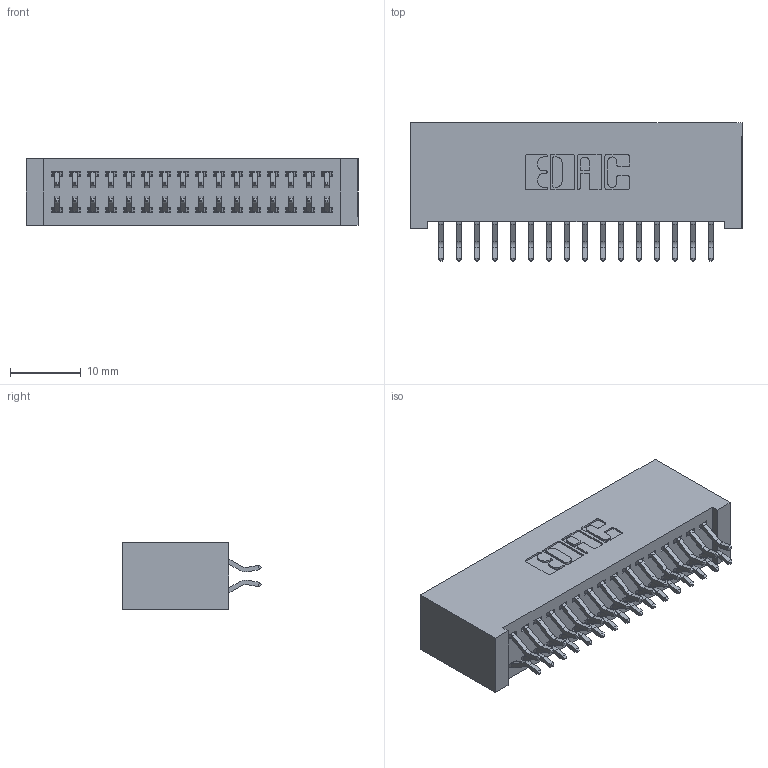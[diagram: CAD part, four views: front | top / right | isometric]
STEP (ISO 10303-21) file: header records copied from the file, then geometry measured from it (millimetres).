
FILE_DESCRIPTION (( 'STEP AP203' ), '1' );
FILE_NAME ('392-032-556-201.STEP', '2019-10-07T14:53:41', ( '' ), ( '' ), 'SwSTEP 2.0', 'SolidWorks 2016', '' );
FILE_SCHEMA (( 'CONFIG_CONTROL_DESIGN' ));
Length unit declared in the file: inch
Products named in the file (3): 392-032-556-201; 342 Part_Lugless; 345-292-001_556 Tail
Assembly tree (33 placements, depth 2):
  392-032-556-201
    342 Part_Lugless
    345-292-001_556 Tail  x32
Bounding box: 46.89 x 19.58 x 9.4 mm (x, y, z)
Volume: 4528.6 mm3; surface area: 7145.9 mm2
Topology: 33 solids, 33 shells, 1958 faces, 5811 edges, 3830 vertices
Faces by surface type: plane 1342, cylinder 616
Entity records: 13467 total; most frequent: CARTESIAN_POINT 2274, ORIENTED_EDGE 2198, DIRECTION 1971, EDGE_CURVE 1099, LINE 971, VECTOR 971, VERTEX_POINT 730, AXIS2_PLACEMENT_3D 500
